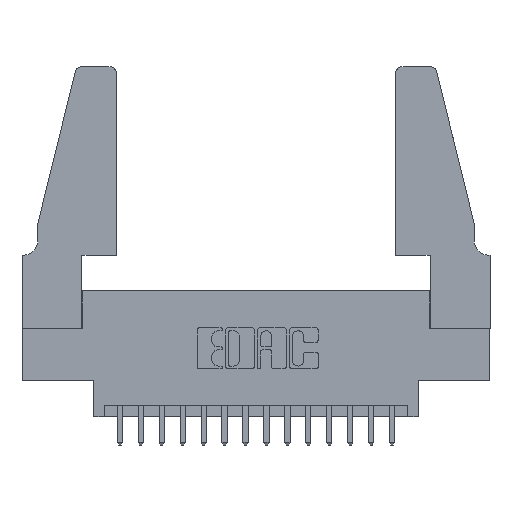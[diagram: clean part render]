
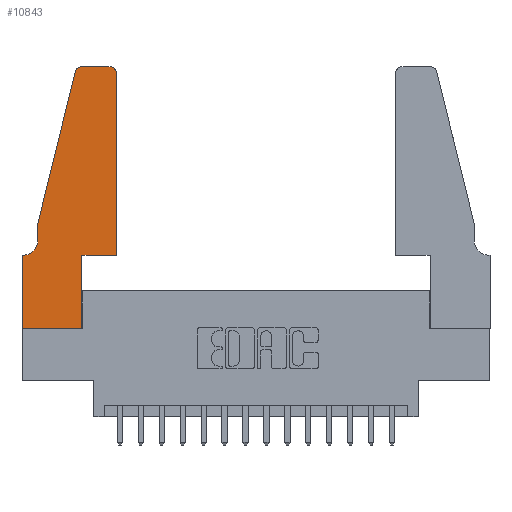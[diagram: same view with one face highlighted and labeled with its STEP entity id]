
A CAD part, top view. The second image highlights one B-rep face of the part: STEP entity #10843.
In plain terms, the highlighted planar face has unit normal (0, 0, 1).
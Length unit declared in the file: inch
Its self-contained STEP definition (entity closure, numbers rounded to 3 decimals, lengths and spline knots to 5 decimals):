
#129 = CARTESIAN_POINT ( 'NONE',  ( 0.0755, 0.5, 0.37 ) ) ;
#218 = CARTESIAN_POINT ( 'NONE',  ( 0.4505, 0.35, 0.37 ) ) ;
#308 = CARTESIAN_POINT ( 'NONE',  ( 0., 0.35, 0.37 ) ) ;
#353 = VECTOR ( 'NONE', #11853, 39.37008 ) ;
#411 = DIRECTION ( 'NONE',  ( 0., 0., 1. ) ) ;
#512 = CARTESIAN_POINT ( 'NONE',  ( 0.2865, 0., 0.37 ) ) ;
#764 = VERTEX_POINT ( 'NONE', #512 ) ;
#948 = VERTEX_POINT ( 'NONE', #129 ) ;
#1261 = EDGE_CURVE ( 'NONE', #12896, #764, #4485, .T. ) ;
#1377 = CARTESIAN_POINT ( 'NONE',  ( 0.25487, 1.22718, 0.37 ) ) ;
#1527 = DIRECTION ( 'NONE',  ( 0., -1., 0. ) ) ;
#1967 = VERTEX_POINT ( 'NONE', #4668 ) ;
#2199 = CARTESIAN_POINT ( 'NONE',  ( 0.4505, 0.35, 0.37 ) ) ;
#2295 = LINE ( 'NONE', #7066, #15762 ) ;
#2371 = AXIS2_PLACEMENT_3D ( 'NONE', #6917, #15881, #8198 ) ;
#2558 = DIRECTION ( 'NONE',  ( 0., 0., 1. ) ) ;
#2598 = CIRCLE ( 'NONE', #13489, 0.07 ) ;
#2973 = EDGE_CURVE ( 'NONE', #4578, #14514, #2295, .T. ) ;
#2992 = DIRECTION ( 'NONE',  ( 0., 1., 0. ) ) ;
#3178 = CARTESIAN_POINT ( 'NONE',  ( 0., 0., 0.37 ) ) ;
#3380 = VECTOR ( 'NONE', #12932, 39.37008 ) ;
#3661 = ORIENTED_EDGE ( 'NONE', *, *, #6874, .T. ) ;
#3798 = CARTESIAN_POINT ( 'NONE',  ( 0.0755, 0.5, 0.37 ) ) ;
#3808 = LINE ( 'NONE', #9023, #3380 ) ;
#3890 = LINE ( 'NONE', #3970, #10444 ) ;
#3949 = ORIENTED_EDGE ( 'NONE', *, *, #11154, .T. ) ;
#3970 = CARTESIAN_POINT ( 'NONE',  ( 0.2605, 1.25, 0.37 ) ) ;
#4375 = VERTEX_POINT ( 'NONE', #12646 ) ;
#4407 = CARTESIAN_POINT ( 'NONE',  ( 0.0055, 0.42, 0.37 ) ) ;
#4485 = LINE ( 'NONE', #3178, #353 ) ;
#4578 = VERTEX_POINT ( 'NONE', #7929 ) ;
#4668 = CARTESIAN_POINT ( 'NONE',  ( 0.0055, 0.35, 0.37 ) ) ;
#4755 = EDGE_CURVE ( 'NONE', #9202, #12896, #14747, .T. ) ;
#4802 = VERTEX_POINT ( 'NONE', #8294 ) ;
#4818 = CARTESIAN_POINT ( 'NONE',  ( 0.2865, 0.35, 0.37 ) ) ;
#5333 = DIRECTION ( 'NONE',  ( -1., 0., 0. ) ) ;
#5409 = VECTOR ( 'NONE', #2992, 39.37008 ) ;
#5418 = ORIENTED_EDGE ( 'NONE', *, *, #16198, .T. ) ;
#5482 = VECTOR ( 'NONE', #16785, 39.37008 ) ;
#5510 = LINE ( 'NONE', #16585, #15390 ) ;
#5586 = EDGE_LOOP ( 'NONE', ( #7301, #15360, #13432, #7866, #9990, #3949, #17087, #6062, #3661, #12166, #5418, #7471 ) ) ;
#5744 = DIRECTION ( 'NONE',  ( -1., 0., 0. ) ) ;
#5756 = AXIS2_PLACEMENT_3D ( 'NONE', #10451, #2558, #11743 ) ;
#5887 = PLANE ( 'NONE',  #14447 ) ;
#5891 = LINE ( 'NONE', #3798, #5482 ) ;
#6062 = ORIENTED_EDGE ( 'NONE', *, *, #1261, .T. ) ;
#6685 = EDGE_CURVE ( 'NONE', #16027, #1967, #2598, .T. ) ;
#6874 = EDGE_CURVE ( 'NONE', #764, #4578, #9409, .T. ) ;
#6917 = CARTESIAN_POINT ( 'NONE',  ( 0.284, 1.22, 0.37 ) ) ;
#7055 = VERTEX_POINT ( 'NONE', #16775 ) ;
#7066 = CARTESIAN_POINT ( 'NONE',  ( 0.4505, 0.35, 0.37 ) ) ;
#7301 = ORIENTED_EDGE ( 'NONE', *, *, #8952, .T. ) ;
#7471 = ORIENTED_EDGE ( 'NONE', *, *, #8287, .T. ) ;
#7491 = VECTOR ( 'NONE', #1527, 39.37008 ) ;
#7866 = ORIENTED_EDGE ( 'NONE', *, *, #11842, .T. ) ;
#7929 = CARTESIAN_POINT ( 'NONE',  ( 0.2865, 0.35, 0.37 ) ) ;
#8190 = CARTESIAN_POINT ( 'NONE',  ( 0., 0., 0.37 ) ) ;
#8198 = DIRECTION ( 'NONE',  ( 1., 0., 0. ) ) ;
#8287 = EDGE_CURVE ( 'NONE', #4375, #4802, #14094, .T. ) ;
#8294 = CARTESIAN_POINT ( 'NONE',  ( 0.4205, 1.25, 0.37 ) ) ;
#8492 = CARTESIAN_POINT ( 'NONE',  ( 0., 0.35, 0.37 ) ) ;
#8851 = LINE ( 'NONE', #218, #5409 ) ;
#8952 = EDGE_CURVE ( 'NONE', #4802, #7055, #3890, .T. ) ;
#8992 = VECTOR ( 'NONE', #10035, 39.37008 ) ;
#9023 = CARTESIAN_POINT ( 'NONE',  ( 0.0755, 0.35, 0.37 ) ) ;
#9202 = VERTEX_POINT ( 'NONE', #308 ) ;
#9409 = LINE ( 'NONE', #4818, #8992 ) ;
#9747 = CIRCLE ( 'NONE', #2371, 0.03 ) ;
#9787 = DIRECTION ( 'NONE',  ( 1., 0., 0. ) ) ;
#9990 = ORIENTED_EDGE ( 'NONE', *, *, #6685, .T. ) ;
#10035 = DIRECTION ( 'NONE',  ( 0., 1., 0. ) ) ;
#10444 = VECTOR ( 'NONE', #5333, 39.37008 ) ;
#10451 = CARTESIAN_POINT ( 'NONE',  ( 0.4205, 1.22, 0.37 ) ) ;
#10843 = ADVANCED_FACE ( 'NONE', ( #15200 ), #5887, .T. ) ;
#11060 = EDGE_CURVE ( 'NONE', #12524, #948, #5510, .T. ) ;
#11154 = EDGE_CURVE ( 'NONE', #1967, #9202, #3808, .T. ) ;
#11389 = EDGE_CURVE ( 'NONE', #7055, #12524, #9747, .T. ) ;
#11683 = DIRECTION ( 'NONE',  ( 1., 0., 0. ) ) ;
#11743 = DIRECTION ( 'NONE',  ( 1., 0., 0. ) ) ;
#11825 = CARTESIAN_POINT ( 'NONE',  ( 0.0755, 0.42, 0.37 ) ) ;
#11842 = EDGE_CURVE ( 'NONE', #948, #16027, #5891, .T. ) ;
#11853 = DIRECTION ( 'NONE',  ( 1., 0., 0. ) ) ;
#12166 = ORIENTED_EDGE ( 'NONE', *, *, #2973, .T. ) ;
#12524 = VERTEX_POINT ( 'NONE', #1377 ) ;
#12599 = CARTESIAN_POINT ( 'NONE',  ( 0., 0., 0.37 ) ) ;
#12646 = CARTESIAN_POINT ( 'NONE',  ( 0.4505, 1.22, 0.37 ) ) ;
#12896 = VERTEX_POINT ( 'NONE', #12599 ) ;
#12932 = DIRECTION ( 'NONE',  ( -1., 0., 0. ) ) ;
#13432 = ORIENTED_EDGE ( 'NONE', *, *, #11060, .T. ) ;
#13455 = DIRECTION ( 'NONE',  ( 0., 0., -1. ) ) ;
#13489 = AXIS2_PLACEMENT_3D ( 'NONE', #4407, #13455, #5744 ) ;
#14094 = CIRCLE ( 'NONE', #5756, 0.03 ) ;
#14447 = AXIS2_PLACEMENT_3D ( 'NONE', #8492, #411, #9787 ) ;
#14514 = VERTEX_POINT ( 'NONE', #2199 ) ;
#14747 = LINE ( 'NONE', #8190, #7491 ) ;
#15200 = FACE_OUTER_BOUND ( 'NONE', #5586, .T. ) ;
#15288 = DIRECTION ( 'NONE',  ( -0.239, -0.971, 0. ) ) ;
#15360 = ORIENTED_EDGE ( 'NONE', *, *, #11389, .T. ) ;
#15390 = VECTOR ( 'NONE', #15288, 39.37008 ) ;
#15762 = VECTOR ( 'NONE', #11683, 39.37008 ) ;
#15881 = DIRECTION ( 'NONE',  ( 0., 0., 1. ) ) ;
#16027 = VERTEX_POINT ( 'NONE', #11825 ) ;
#16198 = EDGE_CURVE ( 'NONE', #14514, #4375, #8851, .T. ) ;
#16585 = CARTESIAN_POINT ( 'NONE',  ( 0.0755, 0.5, 0.37 ) ) ;
#16775 = CARTESIAN_POINT ( 'NONE',  ( 0.284, 1.25, 0.37 ) ) ;
#16785 = DIRECTION ( 'NONE',  ( 0., -1., 0. ) ) ;
#17087 = ORIENTED_EDGE ( 'NONE', *, *, #4755, .T. ) ;
